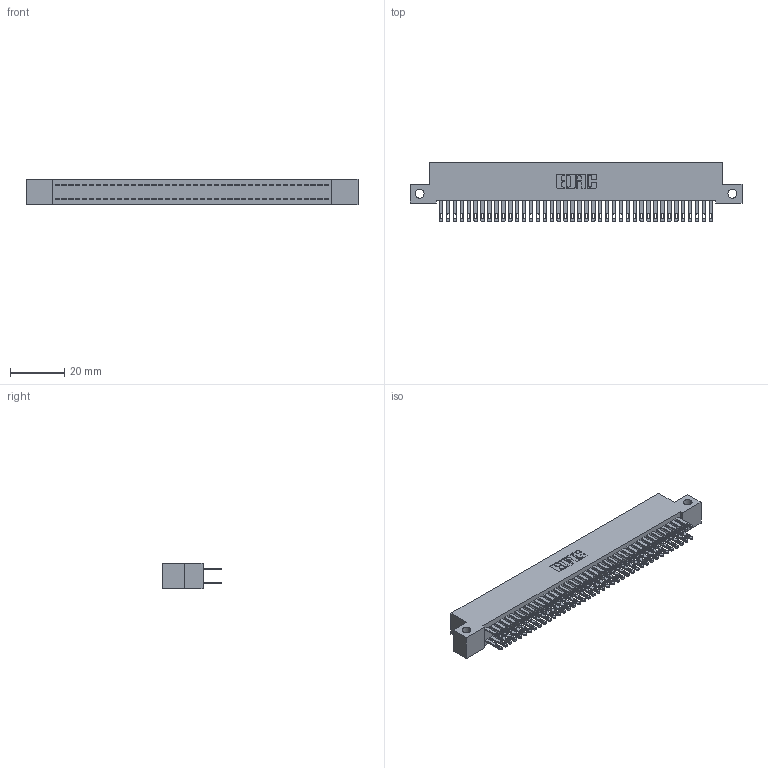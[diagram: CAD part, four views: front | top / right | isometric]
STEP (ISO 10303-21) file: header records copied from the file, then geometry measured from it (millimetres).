
FILE_DESCRIPTION (( 'STEP AP203' ), '1' );
FILE_NAME ('342-080-500-212.STEP', '2019-10-04T11:29:08', ( '' ), ( '' ), 'SwSTEP 2.0', 'SolidWorks 2016', '' );
FILE_SCHEMA (( 'CONFIG_CONTROL_DESIGN' ));
Length unit declared in the file: inch
Products named in the file (3): 345-292-001_345-293-100; 342-080-500-212; 342 Part_Side Mount
Assembly tree (81 placements, depth 2):
  342-080-500-212
    342 Part_Side Mount
    345-292-001_345-293-100  x80
Bounding box: 121.92 x 21.85 x 9.4 mm (x, y, z)
Volume: 11115.6 mm3; surface area: 18650.3 mm2
Topology: 81 solids, 81 shells, 3950 faces, 12059 edges, 8038 vertices
Faces by surface type: plane 2466, cylinder 1484
Entity records: 25793 total; most frequent: CARTESIAN_POINT 4274, ORIENTED_EDGE 4210, DIRECTION 3657, EDGE_CURVE 2105, VECTOR 1973, LINE 1973, VERTEX_POINT 1402, AXIS2_PLACEMENT_3D 842
